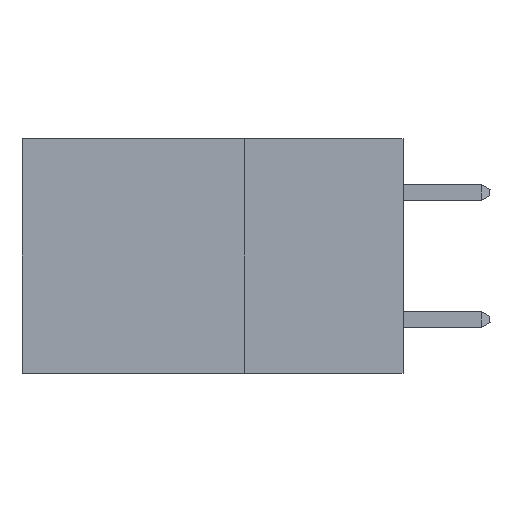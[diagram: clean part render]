
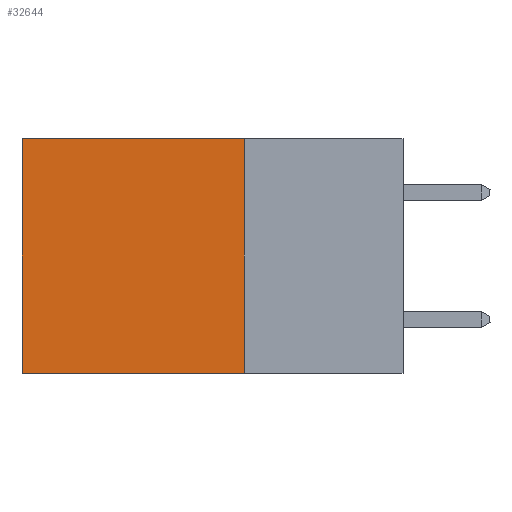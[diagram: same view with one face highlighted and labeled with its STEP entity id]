
A CAD part, left-side view. The second image highlights one B-rep face of the part: STEP entity #32644.
In plain terms, the highlighted planar face has unit normal (-1, 0, 0).
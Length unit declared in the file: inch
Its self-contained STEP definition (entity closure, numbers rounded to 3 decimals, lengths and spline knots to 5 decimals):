
#445 = AXIS2_PLACEMENT_3D ( 'NONE', #710, #15168, #39998 ) ;
#523 = EDGE_LOOP ( 'NONE', ( #10720, #9913, #26706, #1048 ) ) ;
#710 = CARTESIAN_POINT ( 'NONE',  ( 0.2875, 0.25, 0. ) ) ;
#1048 = ORIENTED_EDGE ( 'NONE', *, *, #34266, .T. ) ;
#4836 = VECTOR ( 'NONE', #23729, 39.37008 ) ;
#7711 = DIRECTION ( 'NONE',  ( 0., 1., 0. ) ) ;
#7981 = VERTEX_POINT ( 'NONE', #30502 ) ;
#9913 = ORIENTED_EDGE ( 'NONE', *, *, #36547, .F. ) ;
#10382 = LINE ( 'NONE', #45405, #18685 ) ;
#10720 = ORIENTED_EDGE ( 'NONE', *, *, #40573, .T. ) ;
#12257 = FACE_OUTER_BOUND ( 'NONE', #523, .T. ) ;
#13151 = LINE ( 'NONE', #45008, #4836 ) ;
#15168 = DIRECTION ( 'NONE',  ( 1., 0., 0. ) ) ;
#16530 = VECTOR ( 'NONE', #43192, 39.37008 ) ;
#17638 = LINE ( 'NONE', #28937, #43719 ) ;
#18685 = VECTOR ( 'NONE', #34860, 39.37008 ) ;
#20132 = CARTESIAN_POINT ( 'NONE',  ( 0.2875, 0.25, -0.37 ) ) ;
#22188 = EDGE_CURVE ( 'NONE', #24365, #23189, #35426, .T. ) ;
#23189 = VERTEX_POINT ( 'NONE', #20132 ) ;
#23729 = DIRECTION ( 'NONE',  ( 0., 0., -1. ) ) ;
#24365 = VERTEX_POINT ( 'NONE', #32287 ) ;
#25488 = CARTESIAN_POINT ( 'NONE',  ( 0.2875, 0.25, 0. ) ) ;
#26706 = ORIENTED_EDGE ( 'NONE', *, *, #22188, .F. ) ;
#28937 = CARTESIAN_POINT ( 'NONE',  ( 0.2875, 0.25, 0. ) ) ;
#30502 = CARTESIAN_POINT ( 'NONE',  ( 0.2875, 0.6, -0.37 ) ) ;
#32287 = CARTESIAN_POINT ( 'NONE',  ( 0.2875, 0.25, 0. ) ) ;
#32644 = ADVANCED_FACE ( 'NONE', ( #12257 ), #36435, .F. ) ;
#33916 = CARTESIAN_POINT ( 'NONE',  ( 0.2875, 0.6, 0. ) ) ;
#34266 = EDGE_CURVE ( 'NONE', #24365, #44866, #17638, .T. ) ;
#34860 = DIRECTION ( 'NONE',  ( 0., 1., 0. ) ) ;
#35426 = LINE ( 'NONE', #25488, #16530 ) ;
#36435 = PLANE ( 'NONE',  #445 ) ;
#36547 = EDGE_CURVE ( 'NONE', #23189, #7981, #10382, .T. ) ;
#39998 = DIRECTION ( 'NONE',  ( 0., 0., -1. ) ) ;
#40573 = EDGE_CURVE ( 'NONE', #44866, #7981, #13151, .T. ) ;
#43192 = DIRECTION ( 'NONE',  ( 0., 0., -1. ) ) ;
#43719 = VECTOR ( 'NONE', #7711, 39.37008 ) ;
#44866 = VERTEX_POINT ( 'NONE', #33916 ) ;
#45008 = CARTESIAN_POINT ( 'NONE',  ( 0.2875, 0.6, 0. ) ) ;
#45405 = CARTESIAN_POINT ( 'NONE',  ( 0.2875, 0.25, -0.37 ) ) ;
